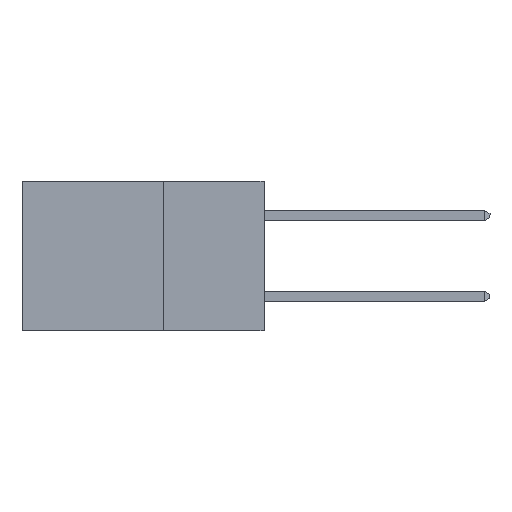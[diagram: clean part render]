
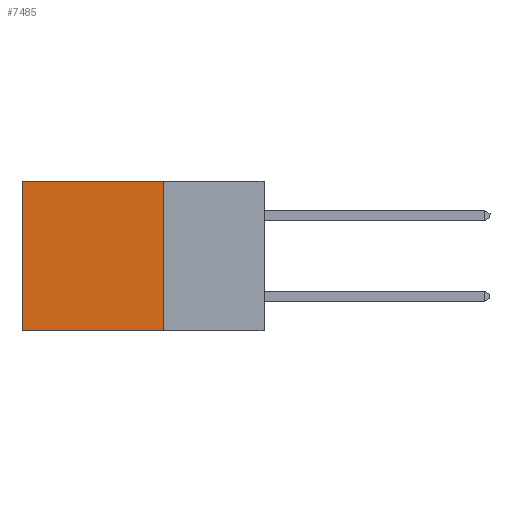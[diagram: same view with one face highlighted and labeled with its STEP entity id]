
A CAD part, left-side view. The second image highlights one B-rep face of the part: STEP entity #7485.
In plain terms, the highlighted planar face has unit normal (-1, 0, 0).
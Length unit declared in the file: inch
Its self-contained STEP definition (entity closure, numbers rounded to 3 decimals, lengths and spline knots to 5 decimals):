
#323 = EDGE_CURVE ( 'NONE', #3709, #17122, #687, .T. ) ;
#687 = LINE ( 'NONE', #7080, #14854 ) ;
#890 = DIRECTION ( 'NONE',  ( 0., 0., -1. ) ) ;
#1034 = CARTESIAN_POINT ( 'NONE',  ( 0.298, 0.25, 0. ) ) ;
#1401 = CARTESIAN_POINT ( 'NONE',  ( 0.298, 0.6, 0. ) ) ;
#1883 = CARTESIAN_POINT ( 'NONE',  ( 0.298, 0.6, 0. ) ) ;
#2070 = EDGE_LOOP ( 'NONE', ( #5736, #5847, #9843, #3089 ) ) ;
#2109 = FACE_OUTER_BOUND ( 'NONE', #2070, .T. ) ;
#2708 = CARTESIAN_POINT ( 'NONE',  ( 0.298, 0.25, -0.37 ) ) ;
#2849 = DIRECTION ( 'NONE',  ( 0., 1., 0. ) ) ;
#3089 = ORIENTED_EDGE ( 'NONE', *, *, #12341, .T. ) ;
#3381 = LINE ( 'NONE', #2708, #7150 ) ;
#3552 = EDGE_CURVE ( 'NONE', #17122, #14799, #3381, .T. ) ;
#3709 = VERTEX_POINT ( 'NONE', #12390 ) ;
#4220 = LINE ( 'NONE', #1883, #14703 ) ;
#5248 = PLANE ( 'NONE',  #10049 ) ;
#5452 = VECTOR ( 'NONE', #15742, 39.37008 ) ;
#5736 = ORIENTED_EDGE ( 'NONE', *, *, #16605, .T. ) ;
#5847 = ORIENTED_EDGE ( 'NONE', *, *, #3552, .F. ) ;
#6666 = DIRECTION ( 'NONE',  ( 0., 0., -1. ) ) ;
#7073 = CARTESIAN_POINT ( 'NONE',  ( 0.298, 0.25, -0.37 ) ) ;
#7080 = CARTESIAN_POINT ( 'NONE',  ( 0.298, 0.25, 0. ) ) ;
#7150 = VECTOR ( 'NONE', #2849, 39.37008 ) ;
#7485 = ADVANCED_FACE ( 'NONE', ( #2109 ), #5248, .F. ) ;
#9843 = ORIENTED_EDGE ( 'NONE', *, *, #323, .F. ) ;
#9996 = VERTEX_POINT ( 'NONE', #1401 ) ;
#10049 = AXIS2_PLACEMENT_3D ( 'NONE', #1034, #14759, #6666 ) ;
#10415 = LINE ( 'NONE', #13120, #5452 ) ;
#10512 = CARTESIAN_POINT ( 'NONE',  ( 0.298, 0.6, -0.37 ) ) ;
#12341 = EDGE_CURVE ( 'NONE', #3709, #9996, #10415, .T. ) ;
#12390 = CARTESIAN_POINT ( 'NONE',  ( 0.298, 0.25, 0. ) ) ;
#12867 = DIRECTION ( 'NONE',  ( 0., 0., -1. ) ) ;
#13120 = CARTESIAN_POINT ( 'NONE',  ( 0.298, 0.25, 0. ) ) ;
#14703 = VECTOR ( 'NONE', #12867, 39.37008 ) ;
#14759 = DIRECTION ( 'NONE',  ( 1., 0., 0. ) ) ;
#14799 = VERTEX_POINT ( 'NONE', #10512 ) ;
#14854 = VECTOR ( 'NONE', #890, 39.37008 ) ;
#15742 = DIRECTION ( 'NONE',  ( 0., 1., 0. ) ) ;
#16605 = EDGE_CURVE ( 'NONE', #9996, #14799, #4220, .T. ) ;
#17122 = VERTEX_POINT ( 'NONE', #7073 ) ;
